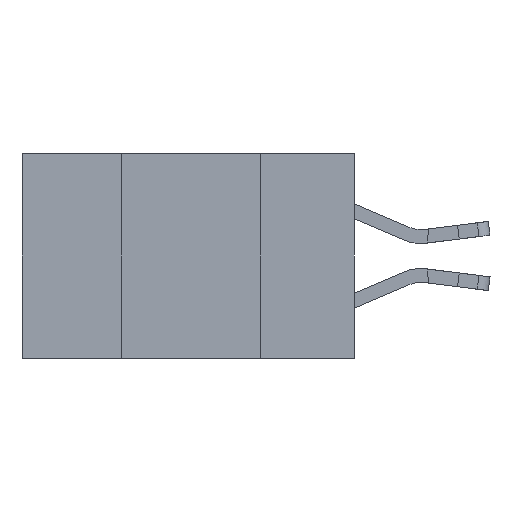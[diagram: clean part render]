
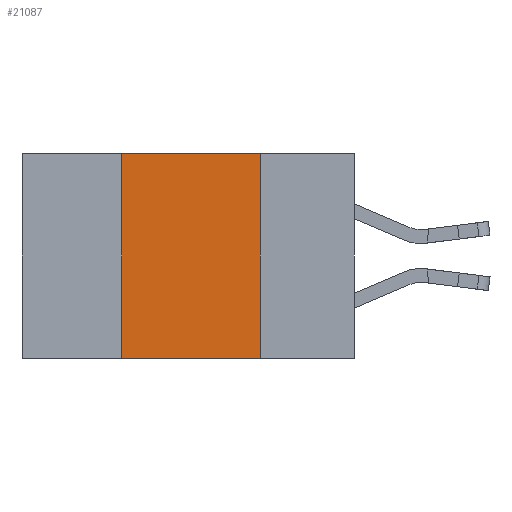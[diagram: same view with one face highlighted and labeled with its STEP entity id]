
A CAD part, left-side view. The second image highlights one B-rep face of the part: STEP entity #21087.
In plain terms, the highlighted planar face has unit normal (-1, 0, 0).
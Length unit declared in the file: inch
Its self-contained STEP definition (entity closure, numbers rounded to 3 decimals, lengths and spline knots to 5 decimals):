
#138 = CARTESIAN_POINT ( 'NONE',  ( 0., 0.42, 0. ) ) ;
#709 = DIRECTION ( 'NONE',  ( 0., -1., 0. ) ) ;
#898 = EDGE_CURVE ( 'NONE', #17925, #11371, #15786, .T. ) ;
#1227 = VECTOR ( 'NONE', #15535, 39.37008 ) ;
#3218 = CARTESIAN_POINT ( 'NONE',  ( 0., 0.42, 0. ) ) ;
#3896 = CARTESIAN_POINT ( 'NONE',  ( 0., 0.6, -0.37 ) ) ;
#3913 = ORIENTED_EDGE ( 'NONE', *, *, #898, .T. ) ;
#4407 = ORIENTED_EDGE ( 'NONE', *, *, #7045, .F. ) ;
#4417 = VERTEX_POINT ( 'NONE', #5077 ) ;
#5077 = CARTESIAN_POINT ( 'NONE',  ( 0., 0.17, 0. ) ) ;
#5423 = LINE ( 'NONE', #138, #1227 ) ;
#7045 = EDGE_CURVE ( 'NONE', #4417, #11371, #11981, .T. ) ;
#7256 = EDGE_CURVE ( 'NONE', #17925, #17356, #5423, .T. ) ;
#10101 = CARTESIAN_POINT ( 'NONE',  ( 0., 0.6, 0. ) ) ;
#10357 = AXIS2_PLACEMENT_3D ( 'NONE', #17078, #18993, #12941 ) ;
#11060 = DIRECTION ( 'NONE',  ( 0., 0., -1. ) ) ;
#11371 = VERTEX_POINT ( 'NONE', #13530 ) ;
#11981 = LINE ( 'NONE', #22428, #18211 ) ;
#12941 = DIRECTION ( 'NONE',  ( 0., 0., -1. ) ) ;
#13297 = FACE_OUTER_BOUND ( 'NONE', #15835, .T. ) ;
#13412 = VECTOR ( 'NONE', #16929, 39.37008 ) ;
#13530 = CARTESIAN_POINT ( 'NONE',  ( 0., 0.17, -0.37 ) ) ;
#14103 = EDGE_CURVE ( 'NONE', #17356, #4417, #22820, .T. ) ;
#14126 = ORIENTED_EDGE ( 'NONE', *, *, #7256, .F. ) ;
#15002 = PLANE ( 'NONE',  #10357 ) ;
#15535 = DIRECTION ( 'NONE',  ( 0., 0., 1. ) ) ;
#15786 = LINE ( 'NONE', #3896, #13412 ) ;
#15835 = EDGE_LOOP ( 'NONE', ( #4407, #21014, #14126, #3913 ) ) ;
#16929 = DIRECTION ( 'NONE',  ( 0., -1., 0. ) ) ;
#17078 = CARTESIAN_POINT ( 'NONE',  ( 0., 0.6, 0. ) ) ;
#17356 = VERTEX_POINT ( 'NONE', #3218 ) ;
#17874 = CARTESIAN_POINT ( 'NONE',  ( 0., 0.42, -0.37 ) ) ;
#17925 = VERTEX_POINT ( 'NONE', #17874 ) ;
#18211 = VECTOR ( 'NONE', #11060, 39.37008 ) ;
#18993 = DIRECTION ( 'NONE',  ( 1., 0., 0. ) ) ;
#21014 = ORIENTED_EDGE ( 'NONE', *, *, #14103, .F. ) ;
#21087 = ADVANCED_FACE ( 'NONE', ( #13297 ), #15002, .F. ) ;
#22247 = VECTOR ( 'NONE', #709, 39.37008 ) ;
#22428 = CARTESIAN_POINT ( 'NONE',  ( 0., 0.17, 0. ) ) ;
#22820 = LINE ( 'NONE', #10101, #22247 ) ;
